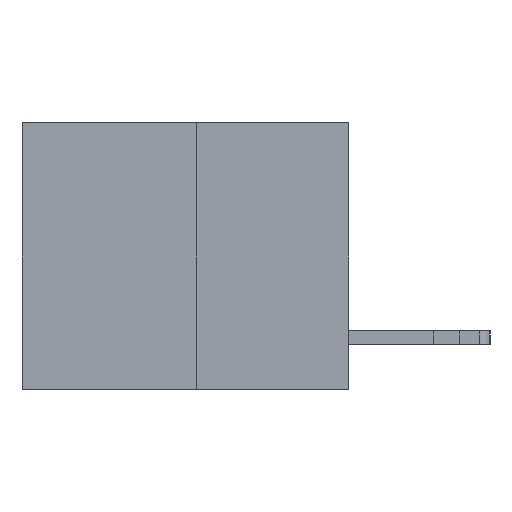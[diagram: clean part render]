
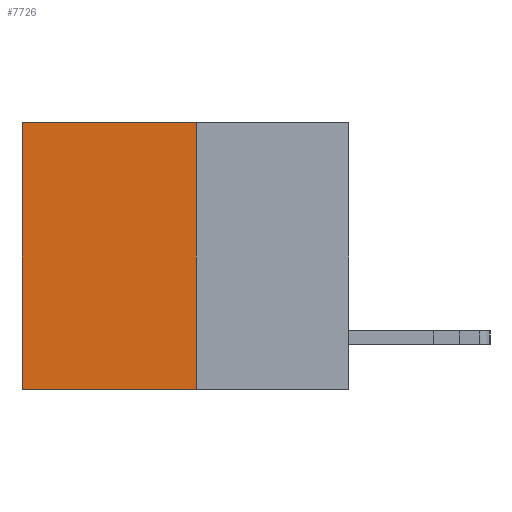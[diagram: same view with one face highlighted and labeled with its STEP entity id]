
A CAD part, left-side view. The second image highlights one B-rep face of the part: STEP entity #7726.
In plain terms, the highlighted planar face has unit normal (-1, 0, 0).
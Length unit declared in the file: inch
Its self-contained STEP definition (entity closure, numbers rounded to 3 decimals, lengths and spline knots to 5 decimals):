
#194 = VERTEX_POINT ( 'NONE', #4533 ) ;
#1170 = ORIENTED_EDGE ( 'NONE', *, *, #10717, .F. ) ;
#1174 = DIRECTION ( 'NONE',  ( 1., 0., 0. ) ) ;
#1361 = CARTESIAN_POINT ( 'NONE',  ( 0.3165, 0.6, 0. ) ) ;
#1441 = VECTOR ( 'NONE', #2257, 39.37008 ) ;
#1778 = FACE_OUTER_BOUND ( 'NONE', #2144, .T. ) ;
#1961 = ORIENTED_EDGE ( 'NONE', *, *, #3901, .F. ) ;
#2144 = EDGE_LOOP ( 'NONE', ( #8937, #1170, #1961, #9382 ) ) ;
#2257 = DIRECTION ( 'NONE',  ( 0., 1., 0. ) ) ;
#2549 = AXIS2_PLACEMENT_3D ( 'NONE', #3989, #1174, #6610 ) ;
#2647 = LINE ( 'NONE', #7997, #8923 ) ;
#2891 = VECTOR ( 'NONE', #12258, 39.37008 ) ;
#3686 = LINE ( 'NONE', #5104, #1441 ) ;
#3899 = VERTEX_POINT ( 'NONE', #7020 ) ;
#3901 = EDGE_CURVE ( 'NONE', #3899, #12516, #2647, .T. ) ;
#3989 = CARTESIAN_POINT ( 'NONE',  ( 0.3165, 0.28, -0.49 ) ) ;
#4027 = VERTEX_POINT ( 'NONE', #1361 ) ;
#4533 = CARTESIAN_POINT ( 'NONE',  ( 0.3165, 0.6, -0.49 ) ) ;
#4555 = LINE ( 'NONE', #11213, #2891 ) ;
#4763 = EDGE_CURVE ( 'NONE', #4027, #194, #8779, .T. ) ;
#4982 = CARTESIAN_POINT ( 'NONE',  ( 0.3165, 0.6, -0.49 ) ) ;
#5104 = CARTESIAN_POINT ( 'NONE',  ( 0.3165, 0.28, 0. ) ) ;
#6610 = DIRECTION ( 'NONE',  ( 0., 0., -1. ) ) ;
#7020 = CARTESIAN_POINT ( 'NONE',  ( 0.3165, 0.28, 0. ) ) ;
#7363 = PLANE ( 'NONE',  #2549 ) ;
#7726 = ADVANCED_FACE ( 'NONE', ( #1778 ), #7363, .F. ) ;
#7997 = CARTESIAN_POINT ( 'NONE',  ( 0.3165, 0.28, -0.49 ) ) ;
#8779 = LINE ( 'NONE', #4982, #11517 ) ;
#8923 = VECTOR ( 'NONE', #12139, 39.37008 ) ;
#8937 = ORIENTED_EDGE ( 'NONE', *, *, #4763, .T. ) ;
#9341 = CARTESIAN_POINT ( 'NONE',  ( 0.3165, 0.28, -0.49 ) ) ;
#9382 = ORIENTED_EDGE ( 'NONE', *, *, #9683, .T. ) ;
#9683 = EDGE_CURVE ( 'NONE', #3899, #4027, #3686, .T. ) ;
#10717 = EDGE_CURVE ( 'NONE', #12516, #194, #4555, .T. ) ;
#11213 = CARTESIAN_POINT ( 'NONE',  ( 0.3165, 0.28, -0.49 ) ) ;
#11517 = VECTOR ( 'NONE', #11852, 39.37008 ) ;
#11852 = DIRECTION ( 'NONE',  ( 0., 0., -1. ) ) ;
#12139 = DIRECTION ( 'NONE',  ( 0., 0., -1. ) ) ;
#12258 = DIRECTION ( 'NONE',  ( 0., 1., 0. ) ) ;
#12516 = VERTEX_POINT ( 'NONE', #9341 ) ;
